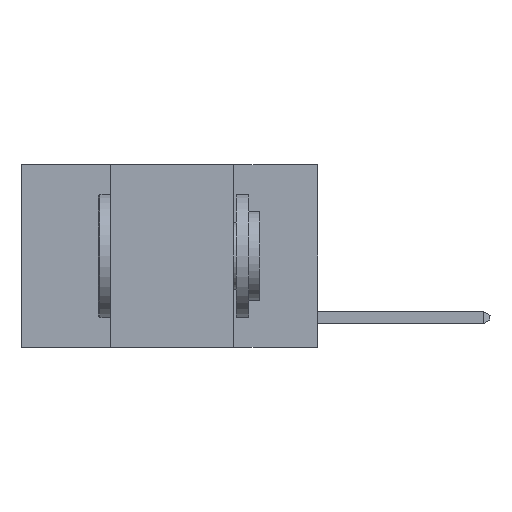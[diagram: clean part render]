
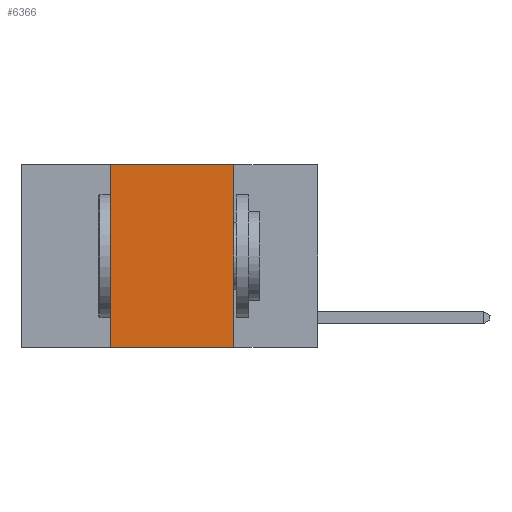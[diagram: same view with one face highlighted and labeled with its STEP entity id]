
A CAD part, left-side view. The second image highlights one B-rep face of the part: STEP entity #6366.
In plain terms, the highlighted planar face has unit normal (-1, 0, 0).
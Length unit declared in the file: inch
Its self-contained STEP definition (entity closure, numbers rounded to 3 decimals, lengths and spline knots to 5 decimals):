
#621 = LINE ( 'NONE', #10078, #11882 ) ;
#630 = PLANE ( 'NONE',  #18856 ) ;
#1541 = ORIENTED_EDGE ( 'NONE', *, *, #9509, .F. ) ;
#2330 = LINE ( 'NONE', #13174, #4548 ) ;
#2879 = DIRECTION ( 'NONE',  ( 1., 0., 0. ) ) ;
#4333 = EDGE_LOOP ( 'NONE', ( #14178, #1541, #22070, #10256 ) ) ;
#4548 = VECTOR ( 'NONE', #17503, 39.37008 ) ;
#4766 = EDGE_CURVE ( 'NONE', #6238, #25997, #18622, .T. ) ;
#5927 = LINE ( 'NONE', #8570, #15745 ) ;
#6238 = VERTEX_POINT ( 'NONE', #19604 ) ;
#6366 = ADVANCED_FACE ( 'NONE', ( #22143 ), #630, .F. ) ;
#8027 = DIRECTION ( 'NONE',  ( 0., 0., 1. ) ) ;
#8570 = CARTESIAN_POINT ( 'NONE',  ( 0., 0.42, 0. ) ) ;
#9509 = EDGE_CURVE ( 'NONE', #17827, #6238, #621, .T. ) ;
#10078 = CARTESIAN_POINT ( 'NONE',  ( 0., 0.6, 0. ) ) ;
#10256 = ORIENTED_EDGE ( 'NONE', *, *, #19141, .T. ) ;
#11882 = VECTOR ( 'NONE', #21337, 39.37008 ) ;
#13174 = CARTESIAN_POINT ( 'NONE',  ( 0., 0.6, -0.37 ) ) ;
#14178 = ORIENTED_EDGE ( 'NONE', *, *, #4766, .F. ) ;
#14888 = CARTESIAN_POINT ( 'NONE',  ( 0., 0.17, -0.37 ) ) ;
#15745 = VECTOR ( 'NONE', #8027, 39.37008 ) ;
#16253 = DIRECTION ( 'NONE',  ( 0., 0., -1. ) ) ;
#17503 = DIRECTION ( 'NONE',  ( 0., -1., 0. ) ) ;
#17749 = CARTESIAN_POINT ( 'NONE',  ( 0., 0.42, 0. ) ) ;
#17827 = VERTEX_POINT ( 'NONE', #17749 ) ;
#18336 = CARTESIAN_POINT ( 'NONE',  ( 0., 0.17, 0. ) ) ;
#18622 = LINE ( 'NONE', #18336, #21548 ) ;
#18856 = AXIS2_PLACEMENT_3D ( 'NONE', #22411, #2879, #20299 ) ;
#19141 = EDGE_CURVE ( 'NONE', #19774, #25997, #2330, .T. ) ;
#19604 = CARTESIAN_POINT ( 'NONE',  ( 0., 0.17, 0. ) ) ;
#19774 = VERTEX_POINT ( 'NONE', #25149 ) ;
#20299 = DIRECTION ( 'NONE',  ( 0., 0., -1. ) ) ;
#21337 = DIRECTION ( 'NONE',  ( 0., -1., 0. ) ) ;
#21548 = VECTOR ( 'NONE', #16253, 39.37008 ) ;
#22070 = ORIENTED_EDGE ( 'NONE', *, *, #25673, .F. ) ;
#22143 = FACE_OUTER_BOUND ( 'NONE', #4333, .T. ) ;
#22411 = CARTESIAN_POINT ( 'NONE',  ( 0., 0.6, 0. ) ) ;
#25149 = CARTESIAN_POINT ( 'NONE',  ( 0., 0.42, -0.37 ) ) ;
#25673 = EDGE_CURVE ( 'NONE', #19774, #17827, #5927, .T. ) ;
#25997 = VERTEX_POINT ( 'NONE', #14888 ) ;
